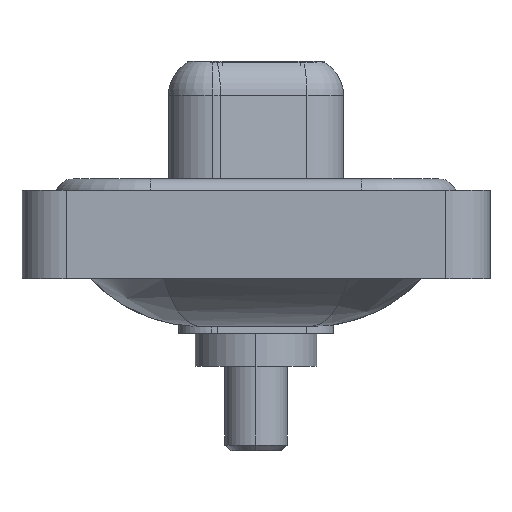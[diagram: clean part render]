
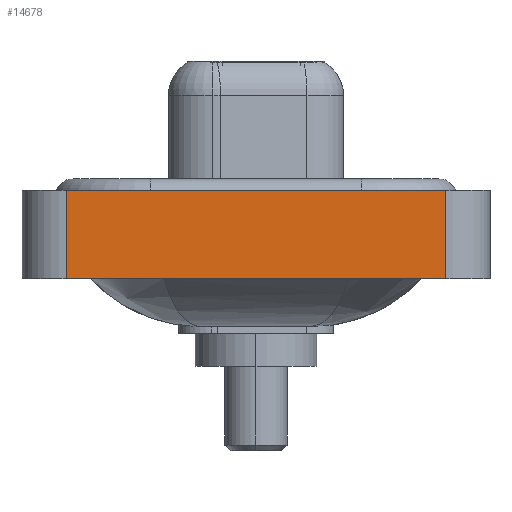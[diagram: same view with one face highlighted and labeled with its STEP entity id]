
A CAD part, left-side view. The second image highlights one B-rep face of the part: STEP entity #14678.
In plain terms, the highlighted planar face has unit normal (-1, 0, 0).
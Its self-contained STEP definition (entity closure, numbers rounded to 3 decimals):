
#362 = CARTESIAN_POINT ( 'NONE',  ( -7.3, -8.55, -3.6 ) ) ;
#1576 = CARTESIAN_POINT ( 'NONE',  ( -7.3, 8.55, -3.6 ) ) ;
#2242 = VERTEX_POINT ( 'NONE', #1576 ) ;
#3233 = ORIENTED_EDGE ( 'NONE', *, *, #8754, .F. ) ;
#3242 = CARTESIAN_POINT ( 'NONE',  ( -7.3, -8.55, -3.6 ) ) ;
#4352 = LINE ( 'NONE', #14679, #4636 ) ;
#4417 = LINE ( 'NONE', #15709, #11228 ) ;
#4582 = VERTEX_POINT ( 'NONE', #14243 ) ;
#4636 = VECTOR ( 'NONE', #9387, 1000. ) ;
#4675 = CARTESIAN_POINT ( 'NONE',  ( -7.3, -8.55, 0.4 ) ) ;
#5888 = ORIENTED_EDGE ( 'NONE', *, *, #15374, .T. ) ;
#5927 = LINE ( 'NONE', #4675, #13840 ) ;
#6560 = VECTOR ( 'NONE', #9394, 1000. ) ;
#7084 = DIRECTION ( 'NONE',  ( 0., -1., 0. ) ) ;
#7183 = EDGE_CURVE ( 'NONE', #2242, #14141, #12884, .T. ) ;
#8121 = EDGE_CURVE ( 'NONE', #10097, #4582, #4417, .T. ) ;
#8754 = EDGE_CURVE ( 'NONE', #14141, #4582, #5927, .T. ) ;
#9208 = ORIENTED_EDGE ( 'NONE', *, *, #8121, .T. ) ;
#9308 = CARTESIAN_POINT ( 'NONE',  ( -7.3, 8.55, -3.6 ) ) ;
#9387 = DIRECTION ( 'NONE',  ( 0., -1., 0. ) ) ;
#9394 = DIRECTION ( 'NONE',  ( 0., 0., 1. ) ) ;
#9397 = AXIS2_PLACEMENT_3D ( 'NONE', #3242, #12004, #15669 ) ;
#9572 = CARTESIAN_POINT ( 'NONE',  ( -7.3, 8.55, 0.4 ) ) ;
#10097 = VERTEX_POINT ( 'NONE', #362 ) ;
#10701 = FACE_OUTER_BOUND ( 'NONE', #15608, .T. ) ;
#11153 = ORIENTED_EDGE ( 'NONE', *, *, #7183, .F. ) ;
#11228 = VECTOR ( 'NONE', #14412, 1000. ) ;
#12004 = DIRECTION ( 'NONE',  ( -1., 0., 0. ) ) ;
#12884 = LINE ( 'NONE', #9308, #6560 ) ;
#13840 = VECTOR ( 'NONE', #7084, 1000. ) ;
#14141 = VERTEX_POINT ( 'NONE', #9572 ) ;
#14243 = CARTESIAN_POINT ( 'NONE',  ( -7.3, -8.55, 0.4 ) ) ;
#14372 = PLANE ( 'NONE',  #9397 ) ;
#14412 = DIRECTION ( 'NONE',  ( 0., 0., 1. ) ) ;
#14678 = ADVANCED_FACE ( 'NONE', ( #10701 ), #14372, .T. ) ;
#14679 = CARTESIAN_POINT ( 'NONE',  ( -7.3, -8.55, -3.6 ) ) ;
#15374 = EDGE_CURVE ( 'NONE', #2242, #10097, #4352, .T. ) ;
#15608 = EDGE_LOOP ( 'NONE', ( #9208, #3233, #11153, #5888 ) ) ;
#15669 = DIRECTION ( 'NONE',  ( 0., 0., 1. ) ) ;
#15709 = CARTESIAN_POINT ( 'NONE',  ( -7.3, -8.55, -3.6 ) ) ;
